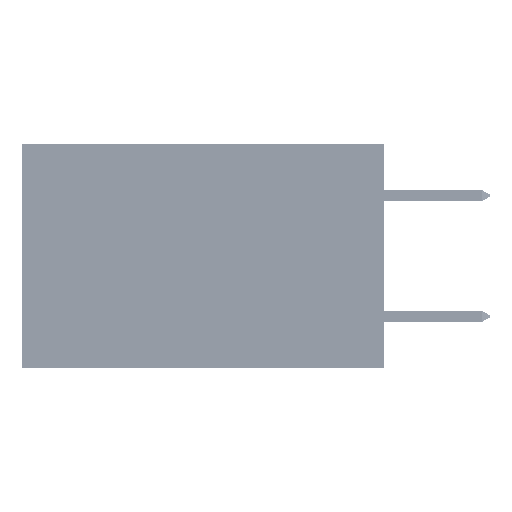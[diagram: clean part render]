
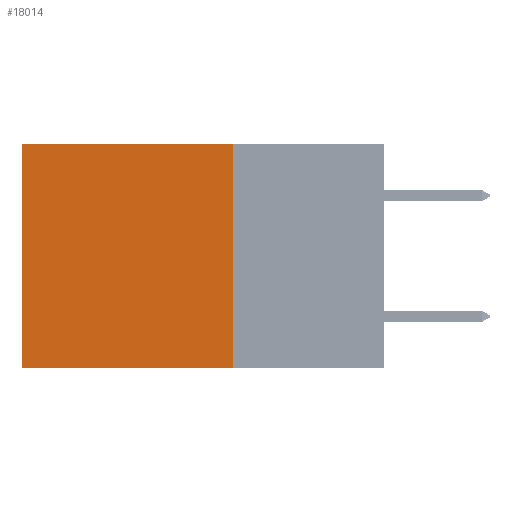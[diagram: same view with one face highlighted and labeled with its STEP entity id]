
A CAD part, left-side view. The second image highlights one B-rep face of the part: STEP entity #18014.
In plain terms, the highlighted planar face has unit normal (-1, 0, 0).
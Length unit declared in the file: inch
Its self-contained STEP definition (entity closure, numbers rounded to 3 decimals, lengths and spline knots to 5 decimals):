
#2948 = ORIENTED_EDGE ( 'NONE', *, *, #21507, .F. ) ;
#3784 = CARTESIAN_POINT ( 'NONE',  ( 0.2875, 0.6, 0. ) ) ;
#5450 = CARTESIAN_POINT ( 'NONE',  ( 0.2875, 0.6, 0. ) ) ;
#6960 = PLANE ( 'NONE',  #33697 ) ;
#7766 = CARTESIAN_POINT ( 'NONE',  ( 0.2875, 0.25, 0. ) ) ;
#8823 = VERTEX_POINT ( 'NONE', #32187 ) ;
#11765 = FACE_OUTER_BOUND ( 'NONE', #26383, .T. ) ;
#14587 = DIRECTION ( 'NONE',  ( 0., 0., -1. ) ) ;
#15485 = EDGE_CURVE ( 'NONE', #8823, #20249, #33339, .T. ) ;
#16363 = DIRECTION ( 'NONE',  ( 0., 0., -1. ) ) ;
#18014 = ADVANCED_FACE ( 'NONE', ( #11765 ), #6960, .F. ) ;
#18366 = LINE ( 'NONE', #38263, #20064 ) ;
#19855 = DIRECTION ( 'NONE',  ( 0., 0., -1. ) ) ;
#20064 = VECTOR ( 'NONE', #19855, 39.37008 ) ;
#20249 = VERTEX_POINT ( 'NONE', #3784 ) ;
#21507 = EDGE_CURVE ( 'NONE', #37245, #31483, #38600, .T. ) ;
#23784 = LINE ( 'NONE', #5450, #39433 ) ;
#24107 = VECTOR ( 'NONE', #35649, 39.37008 ) ;
#24339 = CARTESIAN_POINT ( 'NONE',  ( 0.2875, 0.25, -0.37 ) ) ;
#24816 = ORIENTED_EDGE ( 'NONE', *, *, #32867, .T. ) ;
#26383 = EDGE_LOOP ( 'NONE', ( #24816, #2948, #48038, #30529 ) ) ;
#28055 = CARTESIAN_POINT ( 'NONE',  ( 0.2875, 0.25, 0. ) ) ;
#30529 = ORIENTED_EDGE ( 'NONE', *, *, #15485, .T. ) ;
#31483 = VERTEX_POINT ( 'NONE', #42984 ) ;
#32187 = CARTESIAN_POINT ( 'NONE',  ( 0.2875, 0.25, 0. ) ) ;
#32867 = EDGE_CURVE ( 'NONE', #20249, #31483, #23784, .T. ) ;
#32973 = DIRECTION ( 'NONE',  ( 1., 0., 0. ) ) ;
#33339 = LINE ( 'NONE', #28055, #24107 ) ;
#33697 = AXIS2_PLACEMENT_3D ( 'NONE', #7766, #32973, #14587 ) ;
#34581 = VECTOR ( 'NONE', #36988, 39.37008 ) ;
#35649 = DIRECTION ( 'NONE',  ( 0., 1., 0. ) ) ;
#36228 = EDGE_CURVE ( 'NONE', #8823, #37245, #18366, .T. ) ;
#36988 = DIRECTION ( 'NONE',  ( 0., 1., 0. ) ) ;
#37245 = VERTEX_POINT ( 'NONE', #24339 ) ;
#38263 = CARTESIAN_POINT ( 'NONE',  ( 0.2875, 0.25, 0. ) ) ;
#38600 = LINE ( 'NONE', #41025, #34581 ) ;
#39433 = VECTOR ( 'NONE', #16363, 39.37008 ) ;
#41025 = CARTESIAN_POINT ( 'NONE',  ( 0.2875, 0.25, -0.37 ) ) ;
#42984 = CARTESIAN_POINT ( 'NONE',  ( 0.2875, 0.6, -0.37 ) ) ;
#48038 = ORIENTED_EDGE ( 'NONE', *, *, #36228, .F. ) ;
